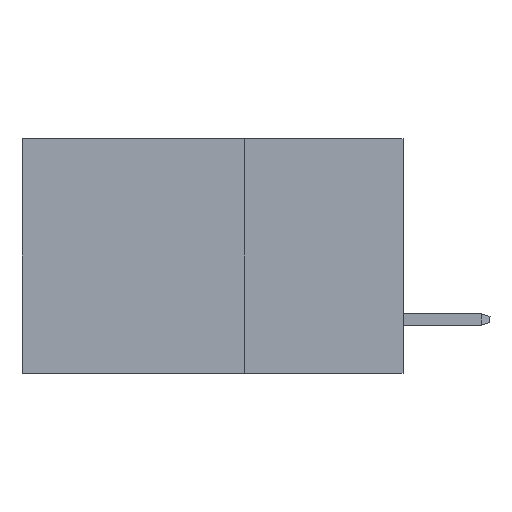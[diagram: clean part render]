
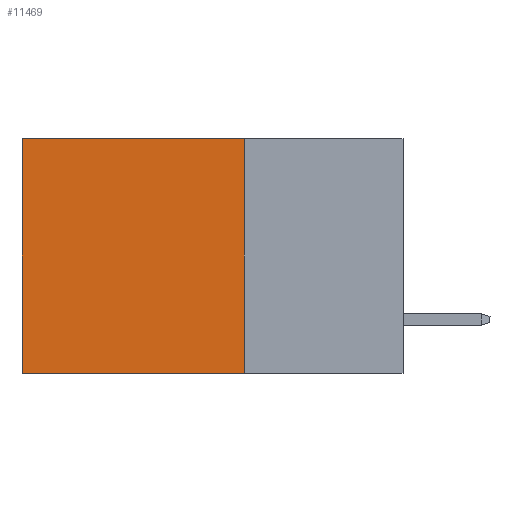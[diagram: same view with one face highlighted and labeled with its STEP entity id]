
A CAD part, left-side view. The second image highlights one B-rep face of the part: STEP entity #11469.
In plain terms, the highlighted planar face has unit normal (-1, 0, 0).
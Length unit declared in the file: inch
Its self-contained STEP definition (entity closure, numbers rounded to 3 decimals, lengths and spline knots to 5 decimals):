
#278 = AXIS2_PLACEMENT_3D ( 'NONE', #8406, #4802, #6491 ) ;
#765 = VECTOR ( 'NONE', #10075, 39.37008 ) ;
#774 = DIRECTION ( 'NONE',  ( 0., 0., -1. ) ) ;
#880 = CARTESIAN_POINT ( 'NONE',  ( 0.2875, 0.25, -0.37 ) ) ;
#1669 = LINE ( 'NONE', #6165, #5571 ) ;
#1964 = EDGE_LOOP ( 'NONE', ( #9076, #6444, #4997, #11196 ) ) ;
#2003 = VECTOR ( 'NONE', #774, 39.37008 ) ;
#2846 = PLANE ( 'NONE',  #278 ) ;
#3253 = VERTEX_POINT ( 'NONE', #7761 ) ;
#3477 = DIRECTION ( 'NONE',  ( 0., 0., -1. ) ) ;
#3498 = CARTESIAN_POINT ( 'NONE',  ( 0.2875, 0.6, 0. ) ) ;
#3506 = VECTOR ( 'NONE', #9901, 39.37008 ) ;
#4578 = EDGE_CURVE ( 'NONE', #9173, #8952, #7207, .T. ) ;
#4802 = DIRECTION ( 'NONE',  ( 1., 0., 0. ) ) ;
#4997 = ORIENTED_EDGE ( 'NONE', *, *, #7228, .F. ) ;
#5571 = VECTOR ( 'NONE', #3477, 39.37008 ) ;
#5989 = VERTEX_POINT ( 'NONE', #880 ) ;
#6165 = CARTESIAN_POINT ( 'NONE',  ( 0.2875, 0.25, 0. ) ) ;
#6444 = ORIENTED_EDGE ( 'NONE', *, *, #7226, .F. ) ;
#6491 = DIRECTION ( 'NONE',  ( 0., 0., -1. ) ) ;
#6548 = FACE_OUTER_BOUND ( 'NONE', #1964, .T. ) ;
#7207 = LINE ( 'NONE', #3498, #2003 ) ;
#7226 = EDGE_CURVE ( 'NONE', #5989, #8952, #10894, .T. ) ;
#7228 = EDGE_CURVE ( 'NONE', #3253, #5989, #1669, .T. ) ;
#7249 = LINE ( 'NONE', #7304, #3506 ) ;
#7304 = CARTESIAN_POINT ( 'NONE',  ( 0.2875, 0.25, 0. ) ) ;
#7761 = CARTESIAN_POINT ( 'NONE',  ( 0.2875, 0.25, 0. ) ) ;
#8406 = CARTESIAN_POINT ( 'NONE',  ( 0.2875, 0.25, 0. ) ) ;
#8685 = EDGE_CURVE ( 'NONE', #3253, #9173, #7249, .T. ) ;
#8952 = VERTEX_POINT ( 'NONE', #9642 ) ;
#9076 = ORIENTED_EDGE ( 'NONE', *, *, #4578, .T. ) ;
#9173 = VERTEX_POINT ( 'NONE', #11254 ) ;
#9642 = CARTESIAN_POINT ( 'NONE',  ( 0.2875, 0.6, -0.37 ) ) ;
#9901 = DIRECTION ( 'NONE',  ( 0., 1., 0. ) ) ;
#10075 = DIRECTION ( 'NONE',  ( 0., 1., 0. ) ) ;
#10778 = CARTESIAN_POINT ( 'NONE',  ( 0.2875, 0.25, -0.37 ) ) ;
#10894 = LINE ( 'NONE', #10778, #765 ) ;
#11196 = ORIENTED_EDGE ( 'NONE', *, *, #8685, .T. ) ;
#11254 = CARTESIAN_POINT ( 'NONE',  ( 0.2875, 0.6, 0. ) ) ;
#11469 = ADVANCED_FACE ( 'NONE', ( #6548 ), #2846, .F. ) ;
